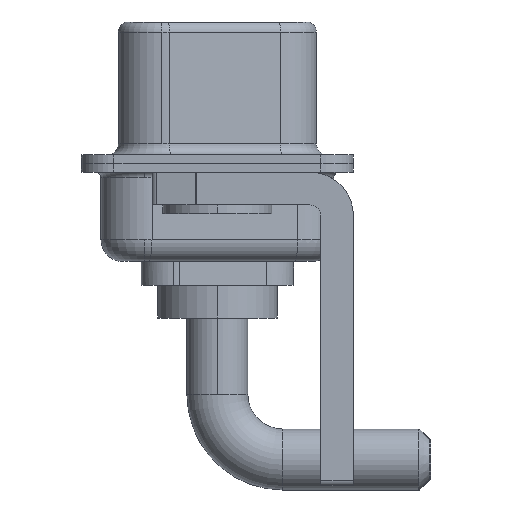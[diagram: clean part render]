
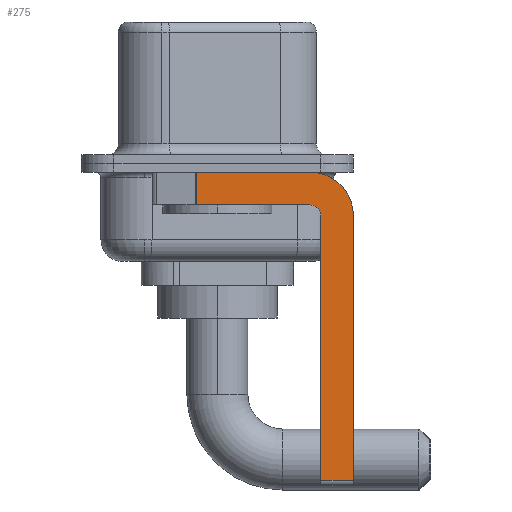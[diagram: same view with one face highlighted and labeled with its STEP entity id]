
A CAD part, left-side view. The second image highlights one B-rep face of the part: STEP entity #275.
In plain terms, the highlighted planar face has unit normal (-1, 0, 0).
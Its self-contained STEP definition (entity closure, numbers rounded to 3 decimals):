
#143 = VERTEX_POINT ( 'NONE', #3964 ) ;
#215 = ORIENTED_EDGE ( 'NONE', *, *, #13794, .F. ) ;
#275 = ADVANCED_FACE ( 'NONE', ( #1738 ), #457, .F. ) ;
#402 = LINE ( 'NONE', #7428, #9641 ) ;
#457 = PLANE ( 'NONE',  #9870 ) ;
#803 = LINE ( 'NONE', #11429, #4945 ) ;
#914 = ORIENTED_EDGE ( 'NONE', *, *, #15038, .T. ) ;
#1367 = VECTOR ( 'NONE', #11725, 1000. ) ;
#1738 = FACE_OUTER_BOUND ( 'NONE', #5598, .T. ) ;
#1956 = CARTESIAN_POINT ( 'NONE',  ( -2.9, 0.978, -1.9 ) ) ;
#2138 = ORIENTED_EDGE ( 'NONE', *, *, #4947, .F. ) ;
#2231 = DIRECTION ( 'NONE',  ( 0., 1., 0. ) ) ;
#2392 = LINE ( 'NONE', #9067, #6186 ) ;
#2725 = DIRECTION ( 'NONE',  ( 0., 0., -1. ) ) ;
#2742 = AXIS2_PLACEMENT_3D ( 'NONE', #11803, #5993, #7140 ) ;
#2845 = CARTESIAN_POINT ( 'NONE',  ( -2.9, -4.25, -2.4 ) ) ;
#2922 = DIRECTION ( 'NONE',  ( -1., 0., 0. ) ) ;
#2995 = DIRECTION ( 'NONE',  ( 0., 0., 1. ) ) ;
#3582 = EDGE_CURVE ( 'NONE', #8020, #143, #2392, .T. ) ;
#3685 = EDGE_CURVE ( 'NONE', #11383, #11722, #13958, .T. ) ;
#3788 = EDGE_CURVE ( 'NONE', #6114, #8020, #14984, .T. ) ;
#3850 = ORIENTED_EDGE ( 'NONE', *, *, #3788, .F. ) ;
#3887 = DIRECTION ( 'NONE',  ( 1., 0., 0. ) ) ;
#3964 = CARTESIAN_POINT ( 'NONE',  ( -2.9, -6.25, -14.55 ) ) ;
#4945 = VECTOR ( 'NONE', #2231, 1000. ) ;
#4947 = EDGE_CURVE ( 'NONE', #5146, #11722, #803, .T. ) ;
#5109 = CARTESIAN_POINT ( 'NONE',  ( -2.9, -4.75, -14.8 ) ) ;
#5146 = VERTEX_POINT ( 'NONE', #7129 ) ;
#5183 = DIRECTION ( 'NONE',  ( 0., 0., 1. ) ) ;
#5345 = AXIS2_PLACEMENT_3D ( 'NONE', #2845, #2922, #2995 ) ;
#5428 = ORIENTED_EDGE ( 'NONE', *, *, #13238, .F. ) ;
#5598 = EDGE_LOOP ( 'NONE', ( #5428, #10310, #2138, #10550, #215, #914, #12835, #3850 ) ) ;
#5993 = DIRECTION ( 'NONE',  ( 1., 0., 0. ) ) ;
#6011 = CARTESIAN_POINT ( 'NONE',  ( -2.9, -6.25, -2.4 ) ) ;
#6114 = VERTEX_POINT ( 'NONE', #9985 ) ;
#6186 = VECTOR ( 'NONE', #7998, 1000. ) ;
#6235 = DIRECTION ( 'NONE',  ( 0., -1., 0. ) ) ;
#6443 = DIRECTION ( 'NONE',  ( 0., -1., 0. ) ) ;
#6974 = VECTOR ( 'NONE', #6235, 1000. ) ;
#7129 = CARTESIAN_POINT ( 'NONE',  ( -2.9, -4.25, -1.9 ) ) ;
#7140 = DIRECTION ( 'NONE',  ( 0., 0., -1. ) ) ;
#7375 = CARTESIAN_POINT ( 'NONE',  ( -2.9, -4.25, -14.55 ) ) ;
#7428 = CARTESIAN_POINT ( 'NONE',  ( -2.9, 3., -0.4 ) ) ;
#7655 = VERTEX_POINT ( 'NONE', #12120 ) ;
#7998 = DIRECTION ( 'NONE',  ( 0., 0., -1. ) ) ;
#8020 = VERTEX_POINT ( 'NONE', #6011 ) ;
#8820 = EDGE_CURVE ( 'NONE', #7655, #5146, #14896, .T. ) ;
#9067 = CARTESIAN_POINT ( 'NONE',  ( -2.9, -6.25, -2.4 ) ) ;
#9641 = VECTOR ( 'NONE', #6443, 1000. ) ;
#9669 = LINE ( 'NONE', #7375, #6974 ) ;
#9870 = AXIS2_PLACEMENT_3D ( 'NONE', #10073, #3887, #2725 ) ;
#9985 = CARTESIAN_POINT ( 'NONE',  ( -2.9, -4.25, -0.4 ) ) ;
#10073 = CARTESIAN_POINT ( 'NONE',  ( -2.9, -4.25, -2.4 ) ) ;
#10310 = ORIENTED_EDGE ( 'NONE', *, *, #3685, .T. ) ;
#10550 = ORIENTED_EDGE ( 'NONE', *, *, #8820, .F. ) ;
#11321 = VERTEX_POINT ( 'NONE', #11930 ) ;
#11383 = VERTEX_POINT ( 'NONE', #12397 ) ;
#11429 = CARTESIAN_POINT ( 'NONE',  ( -2.9, -4.25, -1.9 ) ) ;
#11579 = VECTOR ( 'NONE', #5183, 1000. ) ;
#11722 = VERTEX_POINT ( 'NONE', #1956 ) ;
#11725 = DIRECTION ( 'NONE',  ( 0., 0., -1. ) ) ;
#11803 = CARTESIAN_POINT ( 'NONE',  ( -2.9, -4.25, -2.4 ) ) ;
#11930 = CARTESIAN_POINT ( 'NONE',  ( -2.9, -4.75, -14.55 ) ) ;
#12120 = CARTESIAN_POINT ( 'NONE',  ( -2.9, -4.75, -2.4 ) ) ;
#12397 = CARTESIAN_POINT ( 'NONE',  ( -2.9, 0.978, -0.4 ) ) ;
#12812 = CARTESIAN_POINT ( 'NONE',  ( -2.9, 0.978, -1.9 ) ) ;
#12835 = ORIENTED_EDGE ( 'NONE', *, *, #3582, .F. ) ;
#13238 = EDGE_CURVE ( 'NONE', #11383, #6114, #402, .T. ) ;
#13458 = LINE ( 'NONE', #5109, #11579 ) ;
#13794 = EDGE_CURVE ( 'NONE', #11321, #7655, #13458, .T. ) ;
#13958 = LINE ( 'NONE', #12812, #1367 ) ;
#14896 = CIRCLE ( 'NONE', #5345, 0.5 ) ;
#14984 = CIRCLE ( 'NONE', #2742, 2. ) ;
#15038 = EDGE_CURVE ( 'NONE', #11321, #143, #9669, .T. ) ;
